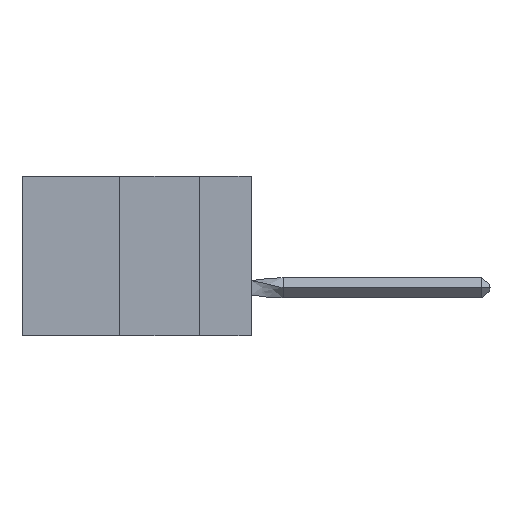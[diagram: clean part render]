
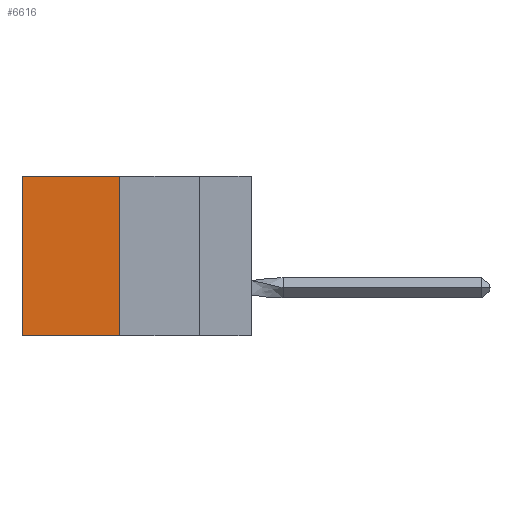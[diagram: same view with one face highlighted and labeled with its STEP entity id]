
A CAD part, left-side view. The second image highlights one B-rep face of the part: STEP entity #6616.
In plain terms, the highlighted planar face has unit normal (-1, 0, 0).
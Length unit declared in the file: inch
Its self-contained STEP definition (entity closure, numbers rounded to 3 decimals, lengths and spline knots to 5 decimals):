
#939 = EDGE_CURVE ( 'NONE', #2826, #11645, #10303, .T. ) ;
#1003 = VECTOR ( 'NONE', #2534, 39.37008 ) ;
#1179 = VERTEX_POINT ( 'NONE', #6230 ) ;
#1184 = ORIENTED_EDGE ( 'NONE', *, *, #4248, .T. ) ;
#1320 = EDGE_CURVE ( 'NONE', #1179, #11645, #13934, .T. ) ;
#2294 = LINE ( 'NONE', #8350, #1003 ) ;
#2534 = DIRECTION ( 'NONE',  ( 0., 1., 0. ) ) ;
#2700 = CARTESIAN_POINT ( 'NONE',  ( 0.305, 0.413, -0.5 ) ) ;
#2826 = VERTEX_POINT ( 'NONE', #8389 ) ;
#3347 = CARTESIAN_POINT ( 'NONE',  ( 0.305, 0.72, -0.5 ) ) ;
#3402 = PLANE ( 'NONE',  #14306 ) ;
#4248 = EDGE_CURVE ( 'NONE', #10731, #1179, #2294, .T. ) ;
#4559 = LINE ( 'NONE', #2700, #12002 ) ;
#5217 = VECTOR ( 'NONE', #8765, 39.37008 ) ;
#5471 = CARTESIAN_POINT ( 'NONE',  ( 0.305, 0.413, -0.5 ) ) ;
#6230 = CARTESIAN_POINT ( 'NONE',  ( 0.305, 0.72, 0. ) ) ;
#6616 = ADVANCED_FACE ( 'NONE', ( #12950 ), #3402, .F. ) ;
#8350 = CARTESIAN_POINT ( 'NONE',  ( 0.305, 0.413, 0. ) ) ;
#8389 = CARTESIAN_POINT ( 'NONE',  ( 0.305, 0.413, -0.5 ) ) ;
#8765 = DIRECTION ( 'NONE',  ( 0., 0., -1. ) ) ;
#9117 = DIRECTION ( 'NONE',  ( 0., 0., -1. ) ) ;
#9781 = CARTESIAN_POINT ( 'NONE',  ( 0.305, 0.72, -0.5 ) ) ;
#10126 = DIRECTION ( 'NONE',  ( 1., 0., 0. ) ) ;
#10303 = LINE ( 'NONE', #5471, #12860 ) ;
#10731 = VERTEX_POINT ( 'NONE', #13968 ) ;
#10977 = ORIENTED_EDGE ( 'NONE', *, *, #13675, .F. ) ;
#11645 = VERTEX_POINT ( 'NONE', #3347 ) ;
#12002 = VECTOR ( 'NONE', #12088, 39.37008 ) ;
#12088 = DIRECTION ( 'NONE',  ( 0., 0., -1. ) ) ;
#12860 = VECTOR ( 'NONE', #13634, 39.37008 ) ;
#12903 = ORIENTED_EDGE ( 'NONE', *, *, #1320, .T. ) ;
#12950 = FACE_OUTER_BOUND ( 'NONE', #13305, .T. ) ;
#13305 = EDGE_LOOP ( 'NONE', ( #12903, #13554, #10977, #1184 ) ) ;
#13554 = ORIENTED_EDGE ( 'NONE', *, *, #939, .F. ) ;
#13634 = DIRECTION ( 'NONE',  ( 0., 1., 0. ) ) ;
#13675 = EDGE_CURVE ( 'NONE', #10731, #2826, #4559, .T. ) ;
#13934 = LINE ( 'NONE', #9781, #5217 ) ;
#13968 = CARTESIAN_POINT ( 'NONE',  ( 0.305, 0.413, 0. ) ) ;
#14306 = AXIS2_PLACEMENT_3D ( 'NONE', #14981, #10126, #9117 ) ;
#14981 = CARTESIAN_POINT ( 'NONE',  ( 0.305, 0.413, -0.5 ) ) ;
